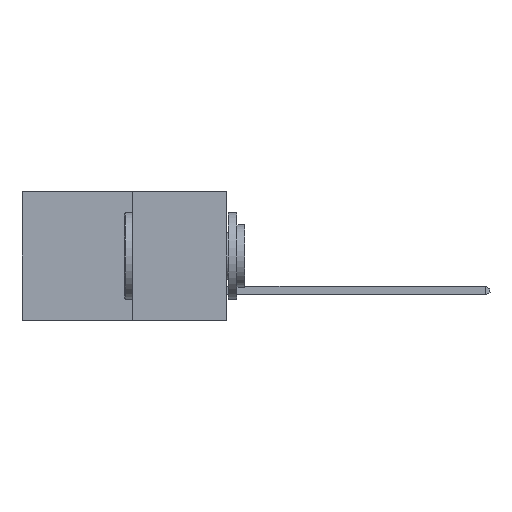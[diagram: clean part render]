
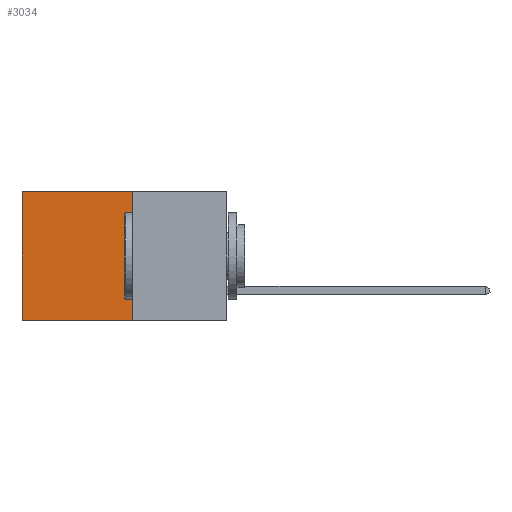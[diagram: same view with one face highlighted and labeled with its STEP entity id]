
A CAD part, left-side view. The second image highlights one B-rep face of the part: STEP entity #3034.
In plain terms, the highlighted planar face has unit normal (-1, 0, 0).
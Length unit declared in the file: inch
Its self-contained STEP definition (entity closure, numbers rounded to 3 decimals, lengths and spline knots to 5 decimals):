
#132 = ORIENTED_EDGE ( 'NONE', *, *, #6097, .T. ) ;
#233 = VECTOR ( 'NONE', #3537, 39.37008 ) ;
#402 = DIRECTION ( 'NONE',  ( 0., 0., -1. ) ) ;
#1114 = DIRECTION ( 'NONE',  ( 0., 0., -1. ) ) ;
#1643 = ORIENTED_EDGE ( 'NONE', *, *, #3212, .F. ) ;
#1703 = LINE ( 'NONE', #4830, #5414 ) ;
#1711 = VECTOR ( 'NONE', #9200, 39.37008 ) ;
#1992 = VERTEX_POINT ( 'NONE', #3567 ) ;
#2720 = DIRECTION ( 'NONE',  ( 1., 0., 0. ) ) ;
#2733 = CARTESIAN_POINT ( 'NONE',  ( 0.277, 0.27, -0.37 ) ) ;
#2936 = ORIENTED_EDGE ( 'NONE', *, *, #8602, .T. ) ;
#3034 = ADVANCED_FACE ( 'NONE', ( #7664 ), #4905, .F. ) ;
#3089 = EDGE_CURVE ( 'NONE', #7459, #1992, #7228, .T. ) ;
#3212 = EDGE_CURVE ( 'NONE', #9078, #7459, #3711, .T. ) ;
#3398 = ORIENTED_EDGE ( 'NONE', *, *, #3089, .F. ) ;
#3462 = CARTESIAN_POINT ( 'NONE',  ( 0.277, 0.27, -0.37 ) ) ;
#3537 = DIRECTION ( 'NONE',  ( 0., 1., 0. ) ) ;
#3567 = CARTESIAN_POINT ( 'NONE',  ( 0.277, 0.59, -0.37 ) ) ;
#3711 = LINE ( 'NONE', #7703, #1711 ) ;
#4219 = CARTESIAN_POINT ( 'NONE',  ( 0.277, 0.27, -0.37 ) ) ;
#4389 = AXIS2_PLACEMENT_3D ( 'NONE', #2733, #2720, #402 ) ;
#4830 = CARTESIAN_POINT ( 'NONE',  ( 0.277, 0.59, -0.37 ) ) ;
#4905 = PLANE ( 'NONE',  #4389 ) ;
#5414 = VECTOR ( 'NONE', #1114, 39.37008 ) ;
#5558 = EDGE_LOOP ( 'NONE', ( #2936, #3398, #1643, #132 ) ) ;
#5705 = CARTESIAN_POINT ( 'NONE',  ( 0.277, 0.27, 0. ) ) ;
#6097 = EDGE_CURVE ( 'NONE', #9078, #8984, #8254, .T. ) ;
#6792 = VECTOR ( 'NONE', #7149, 39.37008 ) ;
#7149 = DIRECTION ( 'NONE',  ( 0., 1., 0. ) ) ;
#7228 = LINE ( 'NONE', #3462, #6792 ) ;
#7434 = CARTESIAN_POINT ( 'NONE',  ( 0.277, 0.59, 0. ) ) ;
#7459 = VERTEX_POINT ( 'NONE', #4219 ) ;
#7558 = CARTESIAN_POINT ( 'NONE',  ( 0.277, 0.27, 0. ) ) ;
#7664 = FACE_OUTER_BOUND ( 'NONE', #5558, .T. ) ;
#7703 = CARTESIAN_POINT ( 'NONE',  ( 0.277, 0.27, -0.37 ) ) ;
#8254 = LINE ( 'NONE', #5705, #233 ) ;
#8602 = EDGE_CURVE ( 'NONE', #8984, #1992, #1703, .T. ) ;
#8984 = VERTEX_POINT ( 'NONE', #7434 ) ;
#9078 = VERTEX_POINT ( 'NONE', #7558 ) ;
#9200 = DIRECTION ( 'NONE',  ( 0., 0., -1. ) ) ;
